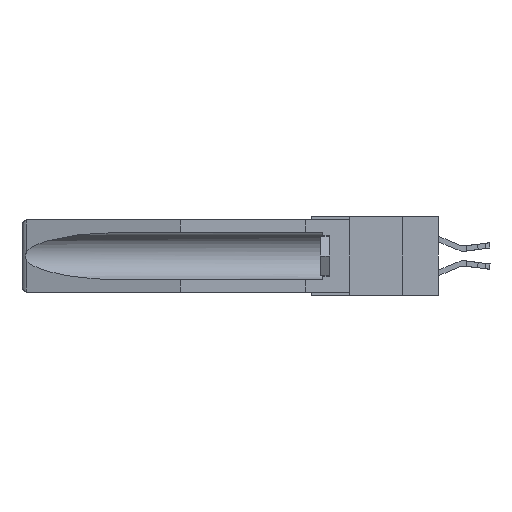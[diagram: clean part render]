
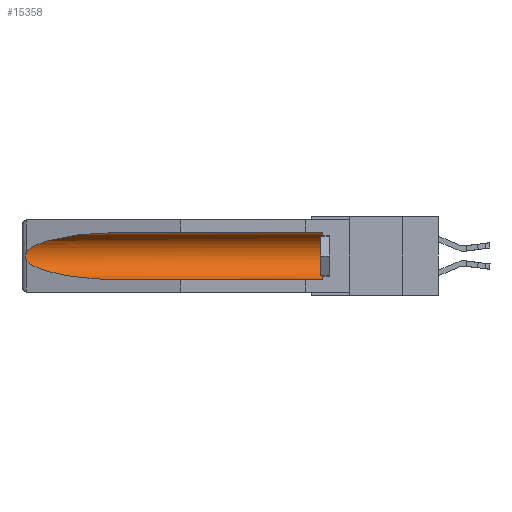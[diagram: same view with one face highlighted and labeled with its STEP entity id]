
A CAD part, left-side view. The second image highlights one B-rep face of the part: STEP entity #15358.
In plain terms, the highlighted cylindrical face has radius 2.857 mm (diameter 5.715 mm), a partial arc.
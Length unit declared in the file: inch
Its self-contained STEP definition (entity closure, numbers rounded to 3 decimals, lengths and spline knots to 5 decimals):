
#34 = CARTESIAN_POINT ( 'NONE',  ( 0.155, 1.07973, -0.284 ) ) ;
#241 = CARTESIAN_POINT ( 'NONE',  ( 0.155, -0.30754, -0.1715 ) ) ;
#623 = FACE_OUTER_BOUND ( 'NONE', #14083, .T. ) ;
#1482 = CARTESIAN_POINT ( 'NONE',  ( 0.26655, 1.53094, -0.18657 ) ) ;
#1841 = CARTESIAN_POINT ( 'NONE',  ( 0.21114, 1.30732, -0.059 ) ) ;
#2731 = ORIENTED_EDGE ( 'NONE', *, *, #11800, .T. ) ;
#3140 = LINE ( 'NONE', #5549, #13734 ) ;
#3291 = CARTESIAN_POINT ( 'NONE',  ( 0.2673, 1.53269, -0.17917 ) ) ;
#4736 = ORIENTED_EDGE ( 'NONE', *, *, #9941, .T. ) ;
#4818 =( BOUNDED_CURVE ( )  B_SPLINE_CURVE ( 3, ( #7937, #1841, #20006, #16022 ),
 .UNSPECIFIED., .F., .F. ) 
 B_SPLINE_CURVE_WITH_KNOTS ( ( 4, 4 ),
 ( 4.71239, 6.08839 ),
 .UNSPECIFIED. ) 
 CURVE ( )  GEOMETRIC_REPRESENTATION_ITEM ( )  RATIONAL_B_SPLINE_CURVE ( ( 1., 0.848, 0.848, 1. ) ) 
 REPRESENTATION_ITEM ( '' )  );
#5129 = AXIS2_PLACEMENT_3D ( 'NONE', #9015, #8935, #12813 ) ;
#5222 = VERTEX_POINT ( 'NONE', #8522 ) ;
#5411 = EDGE_CURVE ( 'NONE', #22696, #7229, #5456, .T. ) ;
#5456 = LINE ( 'NONE', #18506, #11495 ) ;
#5549 = CARTESIAN_POINT ( 'NONE',  ( 0.155, -0.30754, -0.059 ) ) ;
#6712 = CYLINDRICAL_SURFACE ( 'NONE', #10849, 0.1125 ) ;
#7189 = CARTESIAN_POINT ( 'NONE',  ( 0.26537, 1.52718, -0.19328 ) ) ;
#7229 = VERTEX_POINT ( 'NONE', #34 ) ;
#7269 = CARTESIAN_POINT ( 'NONE',  ( 0.26597, 1.52961, -0.15275 ) ) ;
#7937 = CARTESIAN_POINT ( 'NONE',  ( 0.155, 1.07973, -0.059 ) ) ;
#7964 = CARTESIAN_POINT ( 'NONE',  ( 0.25451, 1.48313, -0.24835 ) ) ;
#8168 = ORIENTED_EDGE ( 'NONE', *, *, #11674, .T. ) ;
#8522 = CARTESIAN_POINT ( 'NONE',  ( 0.155, 1.07973, -0.059 ) ) ;
#8935 = DIRECTION ( 'NONE',  ( 0., -1., 0. ) ) ;
#9015 = CARTESIAN_POINT ( 'NONE',  ( 0.155, 0.126, -0.1715 ) ) ;
#9041 = CARTESIAN_POINT ( 'NONE',  ( 0.2675, 1.53308, -0.16763 ) ) ;
#9247 = DIRECTION ( 'NONE',  ( 0., 1., 0. ) ) ;
#9941 = EDGE_CURVE ( 'NONE', #22696, #15730, #14924, .T. ) ;
#10849 = AXIS2_PLACEMENT_3D ( 'NONE', #241, #13813, #15761 ) ;
#10854 = B_SPLINE_CURVE_WITH_KNOTS ( 'NONE', 3,
 ( #14937, #7269, #24653, #12935, #9041, #18683, #3291, #1482, #18767, #7189 ),
 .UNSPECIFIED., .F., .F.,
 ( 4, 2, 2, 2, 4 ),
 ( 0., 0.00029, 0.00058, 0.00087, 0.00117 ),
 .UNSPECIFIED. ) ;
#11495 = VECTOR ( 'NONE', #24385, 39.37008 ) ;
#11621 = CARTESIAN_POINT ( 'NONE',  ( 0.21114, 1.30732, -0.284 ) ) ;
#11674 = EDGE_CURVE ( 'NONE', #5222, #18609, #4818, .T. ) ;
#11800 = EDGE_CURVE ( 'NONE', #13458, #7229, #16426, .T. ) ;
#12813 = DIRECTION ( 'NONE',  ( 0., 0., 1. ) ) ;
#12935 = CARTESIAN_POINT ( 'NONE',  ( 0.2673, 1.5327, -0.16383 ) ) ;
#13458 = VERTEX_POINT ( 'NONE', #14669 ) ;
#13734 = VECTOR ( 'NONE', #9247, 39.37008 ) ;
#13813 = DIRECTION ( 'NONE',  ( 0., 1., 0. ) ) ;
#14083 = EDGE_LOOP ( 'NONE', ( #8168, #19329, #2731, #19875, #4736, #18244 ) ) ;
#14669 = CARTESIAN_POINT ( 'NONE',  ( 0.26537, 1.52718, -0.19328 ) ) ;
#14924 = CIRCLE ( 'NONE', #5129, 0.1125 ) ;
#14937 = CARTESIAN_POINT ( 'NONE',  ( 0.26537, 1.52718, -0.14972 ) ) ;
#15358 = ADVANCED_FACE ( 'NONE', ( #623 ), #6712, .F. ) ;
#15730 = VERTEX_POINT ( 'NONE', #19216 ) ;
#15761 = DIRECTION ( 'NONE',  ( 0., 0., 1. ) ) ;
#16022 = CARTESIAN_POINT ( 'NONE',  ( 0.26537, 1.52718, -0.14972 ) ) ;
#16426 =( BOUNDED_CURVE ( )  B_SPLINE_CURVE ( 3, ( #24785, #7964, #11621, #19377 ),
 .UNSPECIFIED., .F., .F. ) 
 B_SPLINE_CURVE_WITH_KNOTS ( ( 4, 4 ),
 ( 0.1948, 1.5708 ),
 .UNSPECIFIED. ) 
 CURVE ( )  GEOMETRIC_REPRESENTATION_ITEM ( )  RATIONAL_B_SPLINE_CURVE ( ( 1., 0.848, 0.848, 1. ) ) 
 REPRESENTATION_ITEM ( '' )  );
#18244 = ORIENTED_EDGE ( 'NONE', *, *, #24463, .T. ) ;
#18506 = CARTESIAN_POINT ( 'NONE',  ( 0.155, -0.30754, -0.284 ) ) ;
#18609 = VERTEX_POINT ( 'NONE', #19809 ) ;
#18683 = CARTESIAN_POINT ( 'NONE',  ( 0.2675, 1.53308, -0.17534 ) ) ;
#18767 = CARTESIAN_POINT ( 'NONE',  ( 0.26597, 1.5296, -0.19026 ) ) ;
#19216 = CARTESIAN_POINT ( 'NONE',  ( 0.155, 0.126, -0.059 ) ) ;
#19329 = ORIENTED_EDGE ( 'NONE', *, *, #19672, .T. ) ;
#19377 = CARTESIAN_POINT ( 'NONE',  ( 0.155, 1.07973, -0.284 ) ) ;
#19672 = EDGE_CURVE ( 'NONE', #18609, #13458, #10854, .T. ) ;
#19809 = CARTESIAN_POINT ( 'NONE',  ( 0.26537, 1.52718, -0.14972 ) ) ;
#19875 = ORIENTED_EDGE ( 'NONE', *, *, #5411, .F. ) ;
#20006 = CARTESIAN_POINT ( 'NONE',  ( 0.25451, 1.48313, -0.09465 ) ) ;
#22396 = CARTESIAN_POINT ( 'NONE',  ( 0.155, 0.126, -0.284 ) ) ;
#22696 = VERTEX_POINT ( 'NONE', #22396 ) ;
#24385 = DIRECTION ( 'NONE',  ( 0., 1., 0. ) ) ;
#24463 = EDGE_CURVE ( 'NONE', #15730, #5222, #3140, .T. ) ;
#24653 = CARTESIAN_POINT ( 'NONE',  ( 0.26654, 1.53092, -0.15636 ) ) ;
#24785 = CARTESIAN_POINT ( 'NONE',  ( 0.26537, 1.52718, -0.19328 ) ) ;
